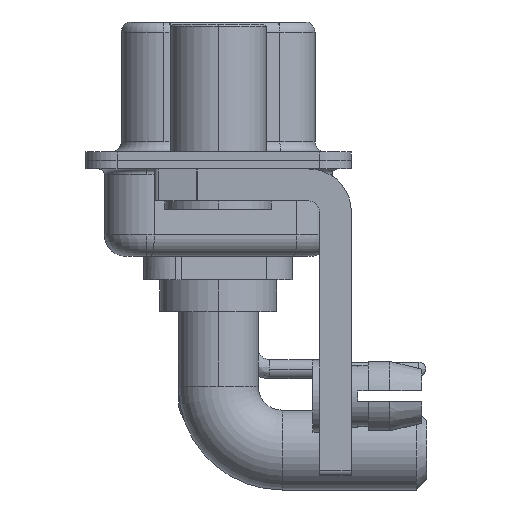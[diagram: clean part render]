
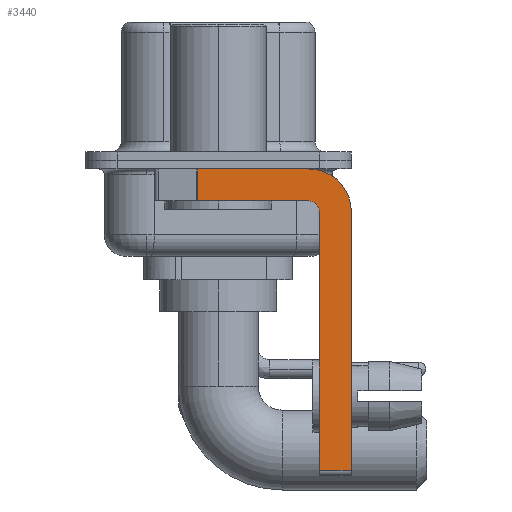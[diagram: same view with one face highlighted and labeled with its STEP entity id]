
A CAD part, left-side view. The second image highlights one B-rep face of the part: STEP entity #3440.
In plain terms, the highlighted planar face has unit normal (-1, 0, 0).
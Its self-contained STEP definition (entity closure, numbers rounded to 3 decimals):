
#8 = EDGE_CURVE ( 'NONE', #5830, #28028, #3165, .T. ) ;
#166 = CIRCLE ( 'NONE', #11223, 0.5 ) ;
#559 = ORIENTED_EDGE ( 'NONE', *, *, #13638, .F. ) ;
#572 = LINE ( 'NONE', #20567, #8588 ) ;
#628 = CARTESIAN_POINT ( 'NONE',  ( -2.9, -4.25, -0.4 ) ) ;
#2366 = CARTESIAN_POINT ( 'NONE',  ( -2.9, -4.75, -2.4 ) ) ;
#3158 = ORIENTED_EDGE ( 'NONE', *, *, #8, .F. ) ;
#3165 = LINE ( 'NONE', #8629, #3524 ) ;
#3327 = DIRECTION ( 'NONE',  ( 0., -1., 0. ) ) ;
#3440 = ADVANCED_FACE ( 'NONE', ( #16767 ), #4031, .F. ) ;
#3524 = VECTOR ( 'NONE', #3327, 1000. ) ;
#3526 = ORIENTED_EDGE ( 'NONE', *, *, #9640, .T. ) ;
#3790 = CARTESIAN_POINT ( 'NONE',  ( -2.9, -6.25, -14.55 ) ) ;
#4031 = PLANE ( 'NONE',  #21180 ) ;
#5383 = EDGE_CURVE ( 'NONE', #32317, #10075, #572, .T. ) ;
#5830 = VERTEX_POINT ( 'NONE', #8468 ) ;
#6793 = VECTOR ( 'NONE', #18576, 1000. ) ;
#6920 = DIRECTION ( 'NONE',  ( 0., 0., -1. ) ) ;
#6968 = ORIENTED_EDGE ( 'NONE', *, *, #19069, .F. ) ;
#7144 = ORIENTED_EDGE ( 'NONE', *, *, #13611, .F. ) ;
#8468 = CARTESIAN_POINT ( 'NONE',  ( -2.9, 0.978, -0.4 ) ) ;
#8588 = VECTOR ( 'NONE', #15609, 1000. ) ;
#8629 = CARTESIAN_POINT ( 'NONE',  ( -2.9, 3., -0.4 ) ) ;
#9640 = EDGE_CURVE ( 'NONE', #5830, #25806, #28341, .T. ) ;
#9830 = CARTESIAN_POINT ( 'NONE',  ( -2.9, -4.25, -1.9 ) ) ;
#10075 = VERTEX_POINT ( 'NONE', #3790 ) ;
#11223 = AXIS2_PLACEMENT_3D ( 'NONE', #16863, #31563, #29764 ) ;
#11468 = CARTESIAN_POINT ( 'NONE',  ( -2.9, -4.25, -2.4 ) ) ;
#11620 = ORIENTED_EDGE ( 'NONE', *, *, #5383, .T. ) ;
#11765 = LINE ( 'NONE', #26974, #17289 ) ;
#11929 = CARTESIAN_POINT ( 'NONE',  ( -2.9, 0.978, -1.9 ) ) ;
#12696 = VERTEX_POINT ( 'NONE', #9830 ) ;
#13611 = EDGE_CURVE ( 'NONE', #32317, #20675, #21640, .T. ) ;
#13638 = EDGE_CURVE ( 'NONE', #20675, #12696, #166, .T. ) ;
#14611 = VECTOR ( 'NONE', #22013, 1000. ) ;
#14712 = DIRECTION ( 'NONE',  ( 0., 0., 1. ) ) ;
#15609 = DIRECTION ( 'NONE',  ( 0., -1., 0. ) ) ;
#16767 = FACE_OUTER_BOUND ( 'NONE', #32358, .T. ) ;
#16863 = CARTESIAN_POINT ( 'NONE',  ( -2.9, -4.25, -2.4 ) ) ;
#16934 = CARTESIAN_POINT ( 'NONE',  ( -2.9, 0.978, -1.9 ) ) ;
#17165 = CARTESIAN_POINT ( 'NONE',  ( -2.9, -6.25, -2.4 ) ) ;
#17289 = VECTOR ( 'NONE', #21837, 1000. ) ;
#18576 = DIRECTION ( 'NONE',  ( 0., 0., -1. ) ) ;
#19069 = EDGE_CURVE ( 'NONE', #22977, #10075, #21847, .T. ) ;
#19248 = ORIENTED_EDGE ( 'NONE', *, *, #30645, .F. ) ;
#19337 = CARTESIAN_POINT ( 'NONE',  ( -2.9, -4.75, -14.8 ) ) ;
#19806 = CARTESIAN_POINT ( 'NONE',  ( -2.9, -4.25, -2.4 ) ) ;
#20479 = ORIENTED_EDGE ( 'NONE', *, *, #23621, .F. ) ;
#20567 = CARTESIAN_POINT ( 'NONE',  ( -2.9, -4.25, -14.55 ) ) ;
#20675 = VERTEX_POINT ( 'NONE', #2366 ) ;
#21180 = AXIS2_PLACEMENT_3D ( 'NONE', #11468, #29168, #29664 ) ;
#21640 = LINE ( 'NONE', #19337, #27078 ) ;
#21837 = DIRECTION ( 'NONE',  ( 0., 1., 0. ) ) ;
#21847 = LINE ( 'NONE', #31937, #14611 ) ;
#22013 = DIRECTION ( 'NONE',  ( 0., 0., -1. ) ) ;
#22977 = VERTEX_POINT ( 'NONE', #17165 ) ;
#23621 = EDGE_CURVE ( 'NONE', #12696, #25806, #11765, .T. ) ;
#23897 = CIRCLE ( 'NONE', #28133, 2. ) ;
#25806 = VERTEX_POINT ( 'NONE', #16934 ) ;
#26974 = CARTESIAN_POINT ( 'NONE',  ( -2.9, -4.25, -1.9 ) ) ;
#27078 = VECTOR ( 'NONE', #14712, 1000. ) ;
#28028 = VERTEX_POINT ( 'NONE', #628 ) ;
#28133 = AXIS2_PLACEMENT_3D ( 'NONE', #19806, #32026, #6920 ) ;
#28341 = LINE ( 'NONE', #11929, #6793 ) ;
#29168 = DIRECTION ( 'NONE',  ( 1., 0., 0. ) ) ;
#29664 = DIRECTION ( 'NONE',  ( 0., 0., -1. ) ) ;
#29758 = CARTESIAN_POINT ( 'NONE',  ( -2.9, -4.75, -14.55 ) ) ;
#29764 = DIRECTION ( 'NONE',  ( 0., 0., 1. ) ) ;
#30645 = EDGE_CURVE ( 'NONE', #28028, #22977, #23897, .T. ) ;
#31563 = DIRECTION ( 'NONE',  ( -1., 0., 0. ) ) ;
#31937 = CARTESIAN_POINT ( 'NONE',  ( -2.9, -6.25, -2.4 ) ) ;
#32026 = DIRECTION ( 'NONE',  ( 1., 0., 0. ) ) ;
#32317 = VERTEX_POINT ( 'NONE', #29758 ) ;
#32358 = EDGE_LOOP ( 'NONE', ( #3158, #3526, #20479, #559, #7144, #11620, #6968, #19248 ) ) ;
